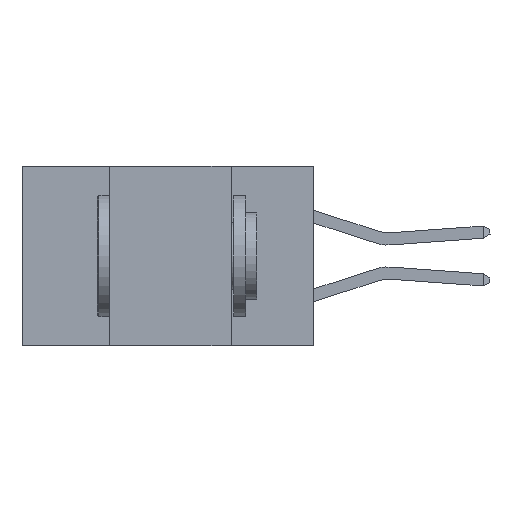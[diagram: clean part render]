
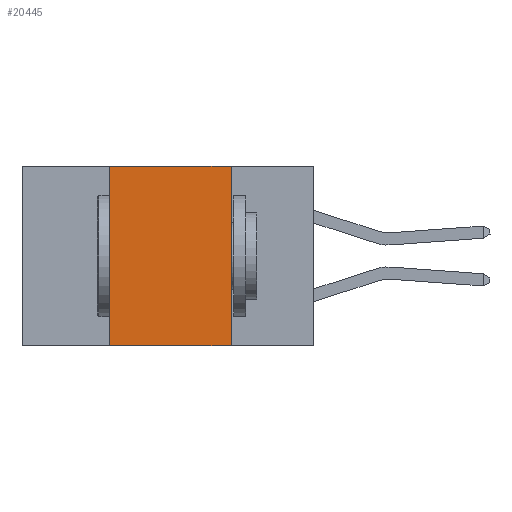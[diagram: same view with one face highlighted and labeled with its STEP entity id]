
A CAD part, left-side view. The second image highlights one B-rep face of the part: STEP entity #20445.
In plain terms, the highlighted planar face has unit normal (-1, 0, 0).
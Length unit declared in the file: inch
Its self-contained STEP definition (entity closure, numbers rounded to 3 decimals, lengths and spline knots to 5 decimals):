
#206 = CARTESIAN_POINT ( 'NONE',  ( 0., 0.6, -0.37 ) ) ;
#353 = LINE ( 'NONE', #18563, #19742 ) ;
#673 = EDGE_CURVE ( 'NONE', #17063, #10561, #3262, .T. ) ;
#2749 = VERTEX_POINT ( 'NONE', #19743 ) ;
#3081 = VECTOR ( 'NONE', #4807, 39.37008 ) ;
#3101 = EDGE_LOOP ( 'NONE', ( #19533, #24406, #3845, #20708 ) ) ;
#3262 = LINE ( 'NONE', #12862, #19907 ) ;
#3845 = ORIENTED_EDGE ( 'NONE', *, *, #673, .F. ) ;
#4678 = EDGE_CURVE ( 'NONE', #10561, #2749, #16930, .T. ) ;
#4807 = DIRECTION ( 'NONE',  ( 0., -1., 0. ) ) ;
#4881 = DIRECTION ( 'NONE',  ( 0., 0., -1. ) ) ;
#5110 = CARTESIAN_POINT ( 'NONE',  ( 0., 0.42, -0.37 ) ) ;
#5391 = VECTOR ( 'NONE', #8767, 39.37008 ) ;
#7509 = VERTEX_POINT ( 'NONE', #22615 ) ;
#7776 = EDGE_CURVE ( 'NONE', #17063, #7509, #17031, .T. ) ;
#8767 = DIRECTION ( 'NONE',  ( 0., -1., 0. ) ) ;
#9134 = CARTESIAN_POINT ( 'NONE',  ( 0., 0.6, 0. ) ) ;
#10561 = VERTEX_POINT ( 'NONE', #24354 ) ;
#11345 = DIRECTION ( 'NONE',  ( 1., 0., 0. ) ) ;
#12436 = EDGE_CURVE ( 'NONE', #2749, #7509, #353, .T. ) ;
#12862 = CARTESIAN_POINT ( 'NONE',  ( 0., 0.42, 0. ) ) ;
#16930 = LINE ( 'NONE', #24929, #5391 ) ;
#17031 = LINE ( 'NONE', #206, #3081 ) ;
#17063 = VERTEX_POINT ( 'NONE', #5110 ) ;
#17895 = PLANE ( 'NONE',  #25661 ) ;
#18563 = CARTESIAN_POINT ( 'NONE',  ( 0., 0.17, 0. ) ) ;
#19533 = ORIENTED_EDGE ( 'NONE', *, *, #12436, .F. ) ;
#19742 = VECTOR ( 'NONE', #23014, 39.37008 ) ;
#19743 = CARTESIAN_POINT ( 'NONE',  ( 0., 0.17, 0. ) ) ;
#19907 = VECTOR ( 'NONE', #23742, 39.37008 ) ;
#20445 = ADVANCED_FACE ( 'NONE', ( #21845 ), #17895, .F. ) ;
#20708 = ORIENTED_EDGE ( 'NONE', *, *, #7776, .T. ) ;
#21845 = FACE_OUTER_BOUND ( 'NONE', #3101, .T. ) ;
#22615 = CARTESIAN_POINT ( 'NONE',  ( 0., 0.17, -0.37 ) ) ;
#23014 = DIRECTION ( 'NONE',  ( 0., 0., -1. ) ) ;
#23742 = DIRECTION ( 'NONE',  ( 0., 0., 1. ) ) ;
#24354 = CARTESIAN_POINT ( 'NONE',  ( 0., 0.42, 0. ) ) ;
#24406 = ORIENTED_EDGE ( 'NONE', *, *, #4678, .F. ) ;
#24929 = CARTESIAN_POINT ( 'NONE',  ( 0., 0.6, 0. ) ) ;
#25661 = AXIS2_PLACEMENT_3D ( 'NONE', #9134, #11345, #4881 ) ;
